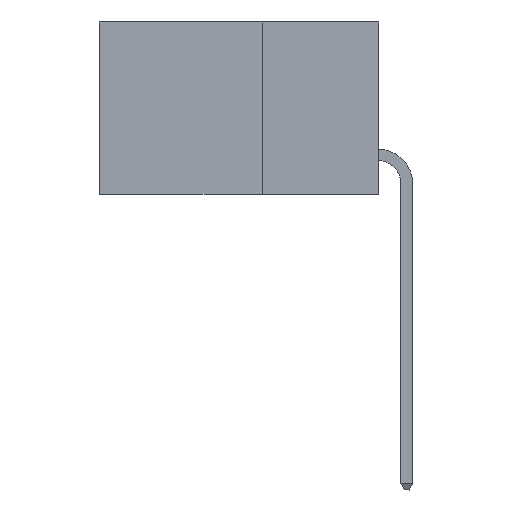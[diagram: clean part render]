
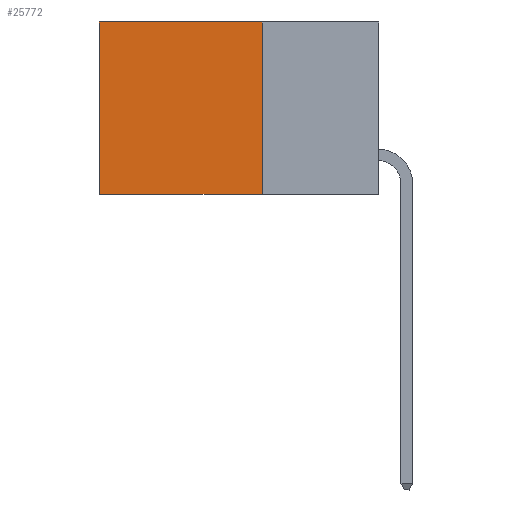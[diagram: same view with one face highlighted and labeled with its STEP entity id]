
A CAD part, left-side view. The second image highlights one B-rep face of the part: STEP entity #25772.
In plain terms, the highlighted planar face has unit normal (-1, 0, 0).
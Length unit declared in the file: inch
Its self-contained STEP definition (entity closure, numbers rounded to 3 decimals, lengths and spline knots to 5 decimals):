
#304 = LINE ( 'NONE', #10937, #11985 ) ;
#320 = VECTOR ( 'NONE', #5961, 39.37008 ) ;
#1527 = CARTESIAN_POINT ( 'NONE',  ( 0.298, 0.25, 0. ) ) ;
#2493 = VERTEX_POINT ( 'NONE', #26148 ) ;
#2603 = LINE ( 'NONE', #26605, #30143 ) ;
#2697 = CARTESIAN_POINT ( 'NONE',  ( 0.298, 0.25, -0.37 ) ) ;
#3483 = EDGE_CURVE ( 'NONE', #2493, #26506, #7338, .T. ) ;
#5961 = DIRECTION ( 'NONE',  ( 0., 1., 0. ) ) ;
#6349 = VERTEX_POINT ( 'NONE', #14254 ) ;
#7338 = LINE ( 'NONE', #2697, #12627 ) ;
#7601 = ORIENTED_EDGE ( 'NONE', *, *, #15961, .F. ) ;
#9949 = ORIENTED_EDGE ( 'NONE', *, *, #21918, .T. ) ;
#9953 = FACE_OUTER_BOUND ( 'NONE', #19060, .T. ) ;
#10937 = CARTESIAN_POINT ( 'NONE',  ( 0.298, 0.25, 0. ) ) ;
#11741 = DIRECTION ( 'NONE',  ( 0., 0., -1. ) ) ;
#11985 = VECTOR ( 'NONE', #18115, 39.37008 ) ;
#12627 = VECTOR ( 'NONE', #19434, 39.37008 ) ;
#13368 = AXIS2_PLACEMENT_3D ( 'NONE', #16999, #24166, #11741 ) ;
#14254 = CARTESIAN_POINT ( 'NONE',  ( 0.298, 0.6, 0. ) ) ;
#15030 = EDGE_CURVE ( 'NONE', #6349, #26506, #2603, .T. ) ;
#15688 = CARTESIAN_POINT ( 'NONE',  ( 0.298, 0.6, -0.37 ) ) ;
#15961 = EDGE_CURVE ( 'NONE', #19429, #2493, #304, .T. ) ;
#16887 = LINE ( 'NONE', #18170, #320 ) ;
#16999 = CARTESIAN_POINT ( 'NONE',  ( 0.298, 0.25, 0. ) ) ;
#18115 = DIRECTION ( 'NONE',  ( 0., 0., -1. ) ) ;
#18170 = CARTESIAN_POINT ( 'NONE',  ( 0.298, 0.25, 0. ) ) ;
#19060 = EDGE_LOOP ( 'NONE', ( #20273, #28088, #7601, #9949 ) ) ;
#19429 = VERTEX_POINT ( 'NONE', #1527 ) ;
#19434 = DIRECTION ( 'NONE',  ( 0., 1., 0. ) ) ;
#20273 = ORIENTED_EDGE ( 'NONE', *, *, #15030, .T. ) ;
#21535 = DIRECTION ( 'NONE',  ( 0., 0., -1. ) ) ;
#21918 = EDGE_CURVE ( 'NONE', #19429, #6349, #16887, .T. ) ;
#24166 = DIRECTION ( 'NONE',  ( 1., 0., 0. ) ) ;
#25772 = ADVANCED_FACE ( 'NONE', ( #9953 ), #31271, .F. ) ;
#26148 = CARTESIAN_POINT ( 'NONE',  ( 0.298, 0.25, -0.37 ) ) ;
#26506 = VERTEX_POINT ( 'NONE', #15688 ) ;
#26605 = CARTESIAN_POINT ( 'NONE',  ( 0.298, 0.6, 0. ) ) ;
#28088 = ORIENTED_EDGE ( 'NONE', *, *, #3483, .F. ) ;
#30143 = VECTOR ( 'NONE', #21535, 39.37008 ) ;
#31271 = PLANE ( 'NONE',  #13368 ) ;
